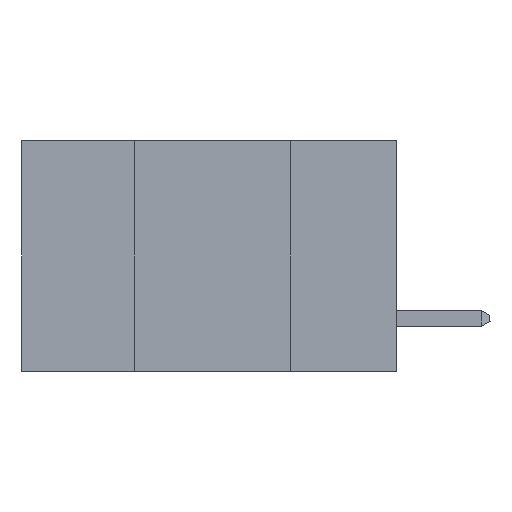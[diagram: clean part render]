
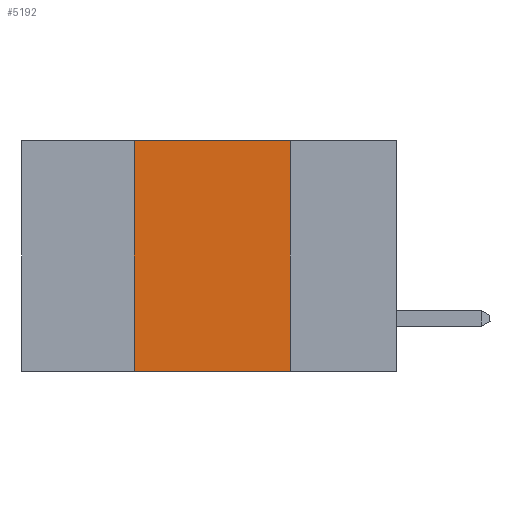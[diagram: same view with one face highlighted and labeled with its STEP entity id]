
A CAD part, left-side view. The second image highlights one B-rep face of the part: STEP entity #5192.
In plain terms, the highlighted planar face has unit normal (-1, 0, 0).
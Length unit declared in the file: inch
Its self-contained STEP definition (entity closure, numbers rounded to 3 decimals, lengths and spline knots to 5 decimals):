
#3 = VECTOR ( 'NONE', #14743, 39.37008 ) ;
#751 = DIRECTION ( 'NONE',  ( 0., -1., 0. ) ) ;
#933 = VERTEX_POINT ( 'NONE', #14346 ) ;
#1737 = EDGE_CURVE ( 'NONE', #10144, #8267, #7110, .T. ) ;
#3325 = LINE ( 'NONE', #5417, #14344 ) ;
#3640 = EDGE_CURVE ( 'NONE', #933, #10144, #3325, .T. ) ;
#3876 = EDGE_CURVE ( 'NONE', #4868, #8267, #10075, .T. ) ;
#3975 = AXIS2_PLACEMENT_3D ( 'NONE', #12801, #6863, #12758 ) ;
#4415 = CARTESIAN_POINT ( 'NONE',  ( 0., 0.17, -0.37 ) ) ;
#4732 = CARTESIAN_POINT ( 'NONE',  ( 0., 0.17, 0. ) ) ;
#4868 = VERTEX_POINT ( 'NONE', #11117 ) ;
#5192 = ADVANCED_FACE ( 'NONE', ( #7212 ), #10478, .F. ) ;
#5417 = CARTESIAN_POINT ( 'NONE',  ( 0., 0.6, 0. ) ) ;
#6114 = CARTESIAN_POINT ( 'NONE',  ( 0., 0.17, 0. ) ) ;
#6752 = ORIENTED_EDGE ( 'NONE', *, *, #3876, .T. ) ;
#6863 = DIRECTION ( 'NONE',  ( 1., 0., 0. ) ) ;
#7055 = VECTOR ( 'NONE', #9881, 39.37008 ) ;
#7110 = LINE ( 'NONE', #6114, #9025 ) ;
#7212 = FACE_OUTER_BOUND ( 'NONE', #10719, .T. ) ;
#7713 = CARTESIAN_POINT ( 'NONE',  ( 0., 0.42, 0. ) ) ;
#8197 = LINE ( 'NONE', #7713, #3 ) ;
#8267 = VERTEX_POINT ( 'NONE', #4415 ) ;
#8692 = CARTESIAN_POINT ( 'NONE',  ( 0., 0.6, -0.37 ) ) ;
#9025 = VECTOR ( 'NONE', #14470, 39.37008 ) ;
#9881 = DIRECTION ( 'NONE',  ( 0., -1., 0. ) ) ;
#10065 = ORIENTED_EDGE ( 'NONE', *, *, #1737, .F. ) ;
#10075 = LINE ( 'NONE', #8692, #7055 ) ;
#10144 = VERTEX_POINT ( 'NONE', #4732 ) ;
#10217 = ORIENTED_EDGE ( 'NONE', *, *, #12033, .F. ) ;
#10478 = PLANE ( 'NONE',  #3975 ) ;
#10719 = EDGE_LOOP ( 'NONE', ( #10065, #14441, #10217, #6752 ) ) ;
#11117 = CARTESIAN_POINT ( 'NONE',  ( 0., 0.42, -0.37 ) ) ;
#12033 = EDGE_CURVE ( 'NONE', #4868, #933, #8197, .T. ) ;
#12758 = DIRECTION ( 'NONE',  ( 0., 0., -1. ) ) ;
#12801 = CARTESIAN_POINT ( 'NONE',  ( 0., 0.6, 0. ) ) ;
#14344 = VECTOR ( 'NONE', #751, 39.37008 ) ;
#14346 = CARTESIAN_POINT ( 'NONE',  ( 0., 0.42, 0. ) ) ;
#14441 = ORIENTED_EDGE ( 'NONE', *, *, #3640, .F. ) ;
#14470 = DIRECTION ( 'NONE',  ( 0., 0., -1. ) ) ;
#14743 = DIRECTION ( 'NONE',  ( 0., 0., 1. ) ) ;
